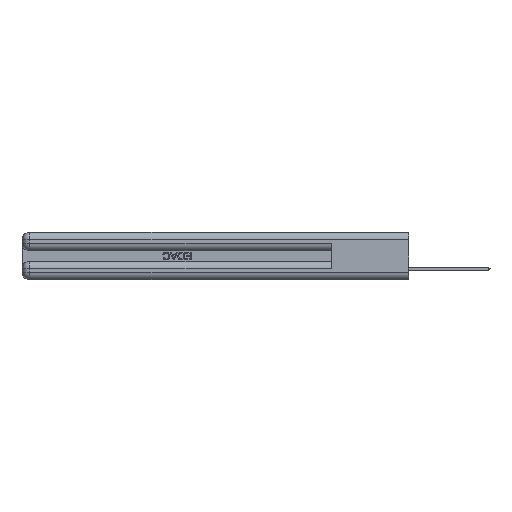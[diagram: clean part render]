
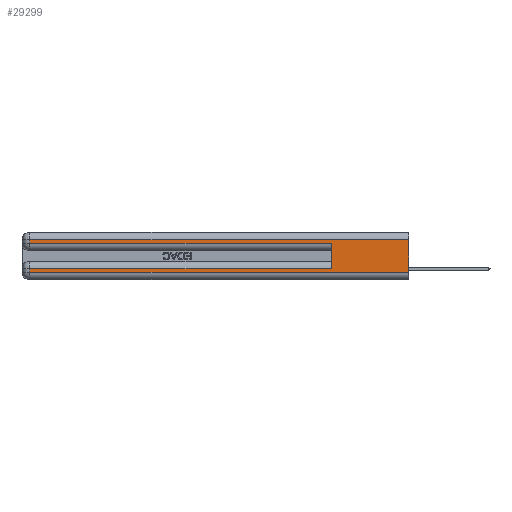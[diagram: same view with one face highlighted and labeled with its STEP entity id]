
A CAD part, left-side view. The second image highlights one B-rep face of the part: STEP entity #29299.
In plain terms, the highlighted planar face has unit normal (-1, 0, 0).
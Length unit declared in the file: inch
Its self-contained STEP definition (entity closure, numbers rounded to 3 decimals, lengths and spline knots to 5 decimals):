
#1349 = DIRECTION ( 'NONE',  ( 0., 0., -1. ) ) ;
#2149 = VERTEX_POINT ( 'NONE', #24064 ) ;
#2604 = EDGE_CURVE ( 'NONE', #21538, #12138, #37240, .T. ) ;
#3140 = EDGE_CURVE ( 'NONE', #45564, #30025, #24356, .T. ) ;
#4129 = VECTOR ( 'NONE', #48019, 39.37008 ) ;
#4448 = LINE ( 'NONE', #36029, #18379 ) ;
#4612 = CARTESIAN_POINT ( 'NONE',  ( 0., 2.94, 0.37 ) ) ;
#5594 = EDGE_CURVE ( 'NONE', #11086, #26728, #27819, .T. ) ;
#5615 = ORIENTED_EDGE ( 'NONE', *, *, #33363, .T. ) ;
#6334 = AXIS2_PLACEMENT_3D ( 'NONE', #13117, #20591, #9207 ) ;
#7599 = VECTOR ( 'NONE', #21087, 39.37008 ) ;
#7930 = CARTESIAN_POINT ( 'NONE',  ( 0., 0., 0.085 ) ) ;
#8514 = VECTOR ( 'NONE', #34349, 39.37008 ) ;
#9207 = DIRECTION ( 'NONE',  ( 0., 0., -1. ) ) ;
#9258 = EDGE_CURVE ( 'NONE', #45217, #45564, #4448, .T. ) ;
#11086 = VERTEX_POINT ( 'NONE', #28517 ) ;
#12138 = VERTEX_POINT ( 'NONE', #25504 ) ;
#13117 = CARTESIAN_POINT ( 'NONE',  ( 0., 0., 0.37 ) ) ;
#13384 = LINE ( 'NONE', #18175, #8514 ) ;
#14026 = ORIENTED_EDGE ( 'NONE', *, *, #2604, .F. ) ;
#17022 = FACE_OUTER_BOUND ( 'NONE', #48713, .T. ) ;
#17393 = VECTOR ( 'NONE', #1349, 39.37008 ) ;
#18175 = CARTESIAN_POINT ( 'NONE',  ( 0., 0., 0.06 ) ) ;
#18321 = DIRECTION ( 'NONE',  ( 0., -1., 0. ) ) ;
#18379 = VECTOR ( 'NONE', #47773, 39.37008 ) ;
#18433 = LINE ( 'NONE', #26892, #40840 ) ;
#18855 = VECTOR ( 'NONE', #18321, 39.37008 ) ;
#18927 = ORIENTED_EDGE ( 'NONE', *, *, #43061, .T. ) ;
#20591 = DIRECTION ( 'NONE',  ( 1., 0., 0. ) ) ;
#21087 = DIRECTION ( 'NONE',  ( 0., 0., 1. ) ) ;
#21538 = VERTEX_POINT ( 'NONE', #40512 ) ;
#21861 = ORIENTED_EDGE ( 'NONE', *, *, #45276, .T. ) ;
#23072 = CARTESIAN_POINT ( 'NONE',  ( 0., 0., 0.285 ) ) ;
#23236 = CARTESIAN_POINT ( 'NONE',  ( 0., 0.6, 0.145 ) ) ;
#23586 = ORIENTED_EDGE ( 'NONE', *, *, #5594, .T. ) ;
#24064 = CARTESIAN_POINT ( 'NONE',  ( 0., 0.6, 0.085 ) ) ;
#24313 = ORIENTED_EDGE ( 'NONE', *, *, #3140, .T. ) ;
#24356 = LINE ( 'NONE', #23072, #18855 ) ;
#25384 = ORIENTED_EDGE ( 'NONE', *, *, #9258, .T. ) ;
#25504 = CARTESIAN_POINT ( 'NONE',  ( 0., 0., 0.06 ) ) ;
#26728 = VERTEX_POINT ( 'NONE', #46436 ) ;
#26729 = DIRECTION ( 'NONE',  ( 0., 1., 0. ) ) ;
#26892 = CARTESIAN_POINT ( 'NONE',  ( 0., 0., 0.31 ) ) ;
#26926 = VECTOR ( 'NONE', #33101, 39.37008 ) ;
#27819 = LINE ( 'NONE', #4612, #17393 ) ;
#28072 = CARTESIAN_POINT ( 'NONE',  ( 0., 2.94, 0.285 ) ) ;
#28517 = CARTESIAN_POINT ( 'NONE',  ( 0., 2.94, 0.085 ) ) ;
#29206 = CARTESIAN_POINT ( 'NONE',  ( 0., 0., 0.37 ) ) ;
#29299 = ADVANCED_FACE ( 'NONE', ( #17022 ), #40185, .F. ) ;
#30025 = VERTEX_POINT ( 'NONE', #45704 ) ;
#33101 = DIRECTION ( 'NONE',  ( 0., 0., -1. ) ) ;
#33363 = EDGE_CURVE ( 'NONE', #2149, #11086, #48454, .T. ) ;
#34349 = DIRECTION ( 'NONE',  ( 0., -1., 0. ) ) ;
#36029 = CARTESIAN_POINT ( 'NONE',  ( 0., 2.94, 0.37 ) ) ;
#37240 = LINE ( 'NONE', #29206, #26926 ) ;
#39860 = EDGE_CURVE ( 'NONE', #2149, #30025, #40444, .T. ) ;
#40185 = PLANE ( 'NONE',  #6334 ) ;
#40444 = LINE ( 'NONE', #23236, #7599 ) ;
#40512 = CARTESIAN_POINT ( 'NONE',  ( 0., 0., 0.31 ) ) ;
#40840 = VECTOR ( 'NONE', #26729, 39.37008 ) ;
#42015 = CARTESIAN_POINT ( 'NONE',  ( 0., 2.94, 0.31 ) ) ;
#43061 = EDGE_CURVE ( 'NONE', #21538, #45217, #18433, .T. ) ;
#45217 = VERTEX_POINT ( 'NONE', #42015 ) ;
#45276 = EDGE_CURVE ( 'NONE', #26728, #12138, #13384, .T. ) ;
#45564 = VERTEX_POINT ( 'NONE', #28072 ) ;
#45695 = ORIENTED_EDGE ( 'NONE', *, *, #39860, .F. ) ;
#45704 = CARTESIAN_POINT ( 'NONE',  ( 0., 0.6, 0.285 ) ) ;
#46436 = CARTESIAN_POINT ( 'NONE',  ( 0., 2.94, 0.06 ) ) ;
#47773 = DIRECTION ( 'NONE',  ( 0., 0., -1. ) ) ;
#48019 = DIRECTION ( 'NONE',  ( 0., 1., 0. ) ) ;
#48454 = LINE ( 'NONE', #7930, #4129 ) ;
#48713 = EDGE_LOOP ( 'NONE', ( #14026, #18927, #25384, #24313, #45695, #5615, #23586, #21861 ) ) ;
